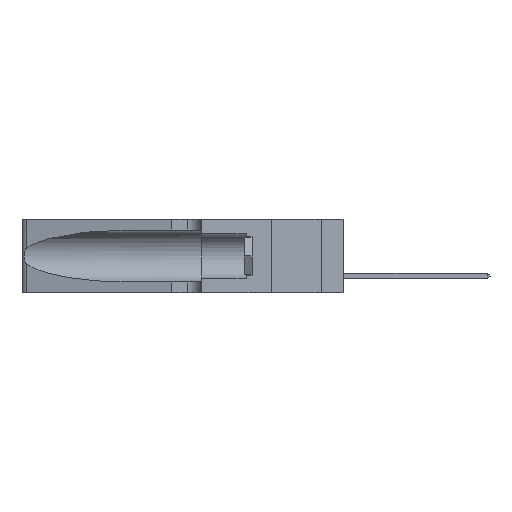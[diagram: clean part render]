
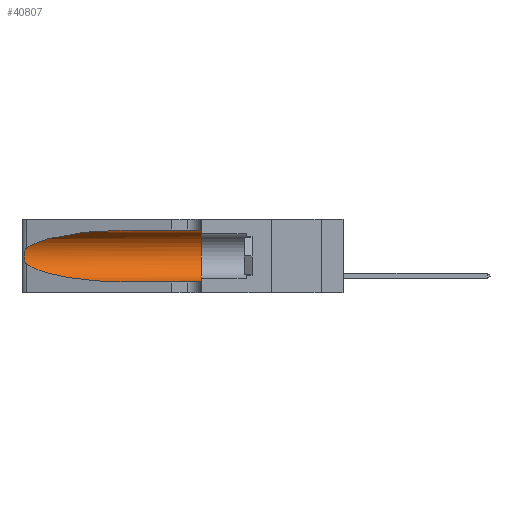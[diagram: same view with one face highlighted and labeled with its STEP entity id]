
A CAD part, left-side view. The second image highlights one B-rep face of the part: STEP entity #40807.
In plain terms, the highlighted cylindrical face has radius 3.308 mm (diameter 6.617 mm), a partial arc.
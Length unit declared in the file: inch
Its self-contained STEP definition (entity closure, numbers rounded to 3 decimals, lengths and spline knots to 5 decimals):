
#48 = EDGE_LOOP ( 'NONE', ( #38823, #37062, #44634, #38394, #42769, #27837 ) ) ;
#321 = CIRCLE ( 'NONE', #43183, 0.13025 ) ;
#644 = VERTEX_POINT ( 'NONE', #20063 ) ;
#3435 = VECTOR ( 'NONE', #34600, 39.37008 ) ;
#6020 = EDGE_CURVE ( 'NONE', #41997, #36792, #34856, .T. ) ;
#6651 = EDGE_CURVE ( 'NONE', #30442, #25792, #34878, .T. ) ;
#8708 = CARTESIAN_POINT ( 'NONE',  ( 0.1305, 1.61858, 0.185 ) ) ;
#9022 = CARTESIAN_POINT ( 'NONE',  ( 0.1305, 1.61858, 0.31525 ) ) ;
#9909 = CARTESIAN_POINT ( 'NONE',  ( 0.1305, 0.72297, 0.31525 ) ) ;
#11441 =( BOUNDED_CURVE ( )  B_SPLINE_CURVE ( 3, ( #45056, #19646, #15840, #30051 ),
 .UNSPECIFIED., .F., .F. ) 
 B_SPLINE_CURVE_WITH_KNOTS ( ( 4, 4 ),
 ( 3.44316, 4.71239 ),
 .UNSPECIFIED. ) 
 CURVE ( )  GEOMETRIC_REPRESENTATION_ITEM ( )  RATIONAL_B_SPLINE_CURVE ( ( 1., 0.87, 0.87, 1. ) ) 
 REPRESENTATION_ITEM ( '' )  );
#11625 = CARTESIAN_POINT ( 'NONE',  ( 0.1305, 0.35, 0.185 ) ) ;
#11677 = CARTESIAN_POINT ( 'NONE',  ( 0.26018, 1.23835, 0.19895 ) ) ;
#12067 = CARTESIAN_POINT ( 'NONE',  ( 0.1305, 1.61858, 0.05475 ) ) ;
#12082 = EDGE_CURVE ( 'NONE', #36792, #30442, #11441, .T. ) ;
#12161 = CARTESIAN_POINT ( 'NONE',  ( 0.25555, 1.22994, 0.2215 ) ) ;
#12781 = AXIS2_PLACEMENT_3D ( 'NONE', #8708, #30753, #41590 ) ;
#13609 = CARTESIAN_POINT ( 'NONE',  ( 0.2373, 1.15595, 0.28018 ) ) ;
#13866 = EDGE_CURVE ( 'NONE', #644, #19847, #18772, .T. ) ;
#14147 = CARTESIAN_POINT ( 'NONE',  ( 0.25487, 1.22718, 0.14631 ) ) ;
#15340 = CARTESIAN_POINT ( 'NONE',  ( 0.25639, 1.23186, 0.15144 ) ) ;
#15840 = CARTESIAN_POINT ( 'NONE',  ( 0.18966, 0.96281, 0.05475 ) ) ;
#17248 = CARTESIAN_POINT ( 'NONE',  ( 0.25487, 1.22718, 0.22369 ) ) ;
#17402 = CARTESIAN_POINT ( 'NONE',  ( 0.18966, 0.96281, 0.31525 ) ) ;
#18772 = LINE ( 'NONE', #9022, #3435 ) ;
#19361 = DIRECTION ( 'NONE',  ( 0., -1., 0. ) ) ;
#19646 = CARTESIAN_POINT ( 'NONE',  ( 0.2373, 1.15595, 0.08982 ) ) ;
#19847 = VERTEX_POINT ( 'NONE', #28012 ) ;
#20063 = CARTESIAN_POINT ( 'NONE',  ( 0.1305, 0.72297, 0.31525 ) ) ;
#20240 = CARTESIAN_POINT ( 'NONE',  ( 0.25487, 1.22718, 0.22369 ) ) ;
#22809 = CARTESIAN_POINT ( 'NONE',  ( 0.25639, 1.23184, 0.21858 ) ) ;
#24291 = EDGE_CURVE ( 'NONE', #644, #41997, #26316, .T. ) ;
#25099 = VECTOR ( 'NONE', #19361, 39.37008 ) ;
#25792 = VERTEX_POINT ( 'NONE', #33797 ) ;
#26316 =( BOUNDED_CURVE ( )  B_SPLINE_CURVE ( 3, ( #9909, #17402, #13609, #17248 ),
 .UNSPECIFIED., .F., .F. ) 
 B_SPLINE_CURVE_WITH_KNOTS ( ( 4, 4 ),
 ( 1.5708, 2.84003 ),
 .UNSPECIFIED. ) 
 CURVE ( )  GEOMETRIC_REPRESENTATION_ITEM ( )  RATIONAL_B_SPLINE_CURVE ( ( 1., 0.87, 0.87, 1. ) ) 
 REPRESENTATION_ITEM ( '' )  );
#27837 = ORIENTED_EDGE ( 'NONE', *, *, #13866, .F. ) ;
#28012 = CARTESIAN_POINT ( 'NONE',  ( 0.1305, 0.35, 0.31525 ) ) ;
#30051 = CARTESIAN_POINT ( 'NONE',  ( 0.1305, 0.72297, 0.05475 ) ) ;
#30360 = CARTESIAN_POINT ( 'NONE',  ( 0.25854, 1.2359, 0.20912 ) ) ;
#30442 = VERTEX_POINT ( 'NONE', #37343 ) ;
#30514 = CARTESIAN_POINT ( 'NONE',  ( 0.25487, 1.22718, 0.22369 ) ) ;
#30675 = CARTESIAN_POINT ( 'NONE',  ( 0.25787, 1.23484, 0.2124 ) ) ;
#30753 = DIRECTION ( 'NONE',  ( 0., -1., 0. ) ) ;
#33647 = DIRECTION ( 'NONE',  ( 0., 1., 0. ) ) ;
#33797 = CARTESIAN_POINT ( 'NONE',  ( 0.1305, 0.35, 0.05475 ) ) ;
#33880 = CARTESIAN_POINT ( 'NONE',  ( 0.26017, 1.23833, 0.17102 ) ) ;
#34600 = DIRECTION ( 'NONE',  ( 0., -1., 0. ) ) ;
#34856 = B_SPLINE_CURVE_WITH_KNOTS ( 'NONE', 3,
 ( #30514, #12161, #22809, #30675, #30360, #11677, #37702, #44556, #33880, #37225, #37382, #15340, #40895, #41509 ),
 .UNSPECIFIED., .F., .F.,
 ( 4, 2, 2, 2, 2, 2, 4 ),
 ( 0., 0.00027, 0.00053, 0.00107, 0.0016, 0.00187, 0.00214 ),
 .UNSPECIFIED. ) ;
#34878 = LINE ( 'NONE', #12067, #25099 ) ;
#36708 = DIRECTION ( 'NONE',  ( 0., 0., 1. ) ) ;
#36792 = VERTEX_POINT ( 'NONE', #14147 ) ;
#37062 = ORIENTED_EDGE ( 'NONE', *, *, #6020, .T. ) ;
#37225 = CARTESIAN_POINT ( 'NONE',  ( 0.25856, 1.23593, 0.16098 ) ) ;
#37343 = CARTESIAN_POINT ( 'NONE',  ( 0.1305, 0.72297, 0.05475 ) ) ;
#37382 = CARTESIAN_POINT ( 'NONE',  ( 0.25789, 1.23486, 0.15765 ) ) ;
#37702 = CARTESIAN_POINT ( 'NONE',  ( 0.26075, 1.23896, 0.19203 ) ) ;
#38394 = ORIENTED_EDGE ( 'NONE', *, *, #6651, .T. ) ;
#38565 = FACE_OUTER_BOUND ( 'NONE', #48, .T. ) ;
#38823 = ORIENTED_EDGE ( 'NONE', *, *, #24291, .T. ) ;
#40807 = ADVANCED_FACE ( 'NONE', ( #38565 ), #47138, .F. ) ;
#40895 = CARTESIAN_POINT ( 'NONE',  ( 0.25555, 1.22993, 0.14849 ) ) ;
#41509 = CARTESIAN_POINT ( 'NONE',  ( 0.25487, 1.22718, 0.14631 ) ) ;
#41590 = DIRECTION ( 'NONE',  ( 0., 0., -1. ) ) ;
#41997 = VERTEX_POINT ( 'NONE', #20240 ) ;
#42769 = ORIENTED_EDGE ( 'NONE', *, *, #45501, .F. ) ;
#43183 = AXIS2_PLACEMENT_3D ( 'NONE', #11625, #33647, #36708 ) ;
#44556 = CARTESIAN_POINT ( 'NONE',  ( 0.26075, 1.23896, 0.178 ) ) ;
#44634 = ORIENTED_EDGE ( 'NONE', *, *, #12082, .T. ) ;
#45056 = CARTESIAN_POINT ( 'NONE',  ( 0.25487, 1.22718, 0.14631 ) ) ;
#45501 = EDGE_CURVE ( 'NONE', #19847, #25792, #321, .T. ) ;
#47138 = CYLINDRICAL_SURFACE ( 'NONE', #12781, 0.13025 ) ;
